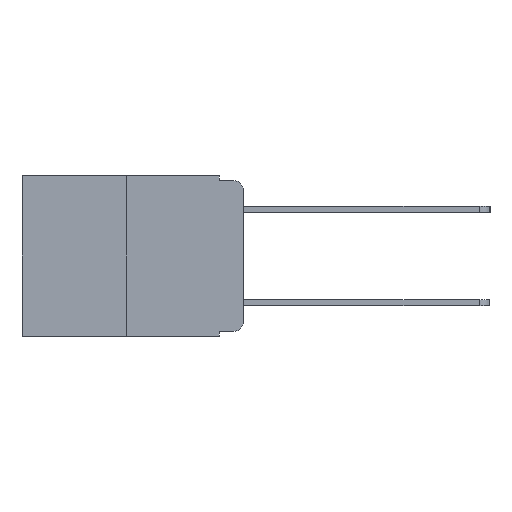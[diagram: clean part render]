
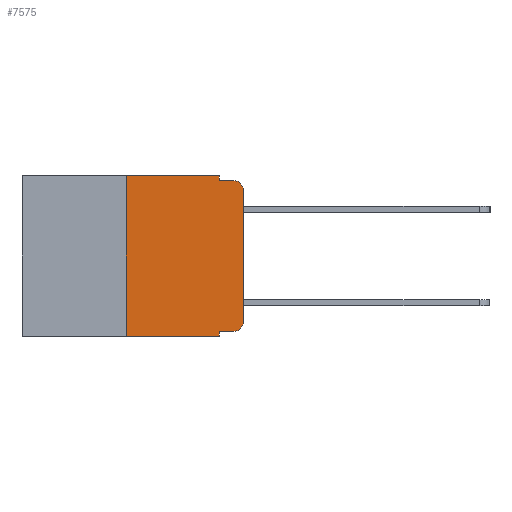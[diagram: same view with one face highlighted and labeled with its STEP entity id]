
A CAD part, left-side view. The second image highlights one B-rep face of the part: STEP entity #7575.
In plain terms, the highlighted planar face has unit normal (-1, 0, 0).
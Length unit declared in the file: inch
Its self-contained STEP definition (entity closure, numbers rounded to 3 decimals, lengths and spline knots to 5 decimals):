
#21 = ORIENTED_EDGE ( 'NONE', *, *, #9780, .F. ) ;
#53 = EDGE_CURVE ( 'NONE', #6673, #9982, #2832, .T. ) ;
#130 = VERTEX_POINT ( 'NONE', #5773 ) ;
#271 = DIRECTION ( 'NONE',  ( 0., 0., 1. ) ) ;
#294 = PLANE ( 'NONE',  #10442 ) ;
#324 = LINE ( 'NONE', #3387, #2792 ) ;
#1171 = DIRECTION ( 'NONE',  ( -1., 0., 0. ) ) ;
#1181 = CARTESIAN_POINT ( 'NONE',  ( 0., 0.02, -0.01 ) ) ;
#1398 = CARTESIAN_POINT ( 'NONE',  ( 0., 0.473, 0. ) ) ;
#1444 = DIRECTION ( 'NONE',  ( 0., 0., -1. ) ) ;
#1502 = CARTESIAN_POINT ( 'NONE',  ( 0., 0.051, -0.343 ) ) ;
#1526 = CARTESIAN_POINT ( 'NONE',  ( 0., 0.25, -0.343 ) ) ;
#1601 = VERTEX_POINT ( 'NONE', #10318 ) ;
#1723 = CARTESIAN_POINT ( 'NONE',  ( 0., 0., -0.313 ) ) ;
#2147 = AXIS2_PLACEMENT_3D ( 'NONE', #6851, #1171, #7711 ) ;
#2165 = CARTESIAN_POINT ( 'NONE',  ( 0., 0.02, -0.313 ) ) ;
#2290 = VECTOR ( 'NONE', #9321, 39.37008 ) ;
#2334 = VERTEX_POINT ( 'NONE', #5200 ) ;
#2429 = DIRECTION ( 'NONE',  ( 0., 0., -1. ) ) ;
#2653 = FACE_OUTER_BOUND ( 'NONE', #3394, .T. ) ;
#2792 = VECTOR ( 'NONE', #271, 39.37008 ) ;
#2832 = LINE ( 'NONE', #11285, #3919 ) ;
#2994 = ORIENTED_EDGE ( 'NONE', *, *, #10386, .T. ) ;
#3154 = DIRECTION ( 'NONE',  ( 0., 0., -1. ) ) ;
#3289 = ORIENTED_EDGE ( 'NONE', *, *, #9850, .T. ) ;
#3387 = CARTESIAN_POINT ( 'NONE',  ( 0., 0.25, 0. ) ) ;
#3394 = EDGE_LOOP ( 'NONE', ( #2994, #3289, #6341, #8844, #21, #4039, #3494, #9813, #10316, #4679 ) ) ;
#3494 = ORIENTED_EDGE ( 'NONE', *, *, #53, .T. ) ;
#3524 = VERTEX_POINT ( 'NONE', #8929 ) ;
#3849 = CARTESIAN_POINT ( 'NONE',  ( 0., 0.473, 0. ) ) ;
#3919 = VECTOR ( 'NONE', #10484, 39.37008 ) ;
#3980 = CARTESIAN_POINT ( 'NONE',  ( 0., 0., 0. ) ) ;
#4039 = ORIENTED_EDGE ( 'NONE', *, *, #8185, .F. ) ;
#4239 = LINE ( 'NONE', #3849, #6384 ) ;
#4679 = ORIENTED_EDGE ( 'NONE', *, *, #6466, .T. ) ;
#4829 = LINE ( 'NONE', #10933, #2290 ) ;
#4880 = VERTEX_POINT ( 'NONE', #11084 ) ;
#4928 = VECTOR ( 'NONE', #11630, 39.37008 ) ;
#5101 = CARTESIAN_POINT ( 'NONE',  ( 0., 0.051, 0. ) ) ;
#5200 = CARTESIAN_POINT ( 'NONE',  ( 0., 0., -0.03 ) ) ;
#5322 = CIRCLE ( 'NONE', #6218, 0.02 ) ;
#5773 = CARTESIAN_POINT ( 'NONE',  ( 0., 0.051, -0.333 ) ) ;
#5828 = CIRCLE ( 'NONE', #2147, 0.02 ) ;
#6218 = AXIS2_PLACEMENT_3D ( 'NONE', #2165, #8504, #3154 ) ;
#6258 = VECTOR ( 'NONE', #8592, 39.37008 ) ;
#6310 = LINE ( 'NONE', #10522, #8564 ) ;
#6341 = ORIENTED_EDGE ( 'NONE', *, *, #9297, .F. ) ;
#6384 = VECTOR ( 'NONE', #10751, 39.37008 ) ;
#6466 = EDGE_CURVE ( 'NONE', #3524, #7777, #5322, .T. ) ;
#6673 = VERTEX_POINT ( 'NONE', #1526 ) ;
#6851 = CARTESIAN_POINT ( 'NONE',  ( 0., 0.02, -0.03 ) ) ;
#7059 = EDGE_CURVE ( 'NONE', #130, #3524, #6310, .T. ) ;
#7344 = LINE ( 'NONE', #3980, #4928 ) ;
#7575 = ADVANCED_FACE ( 'NONE', ( #2653 ), #294, .F. ) ;
#7630 = EDGE_CURVE ( 'NONE', #130, #9982, #11343, .T. ) ;
#7711 = DIRECTION ( 'NONE',  ( 0., 0., -1. ) ) ;
#7777 = VERTEX_POINT ( 'NONE', #1723 ) ;
#7889 = DIRECTION ( 'NONE',  ( 1., 0., 0. ) ) ;
#8185 = EDGE_CURVE ( 'NONE', #6673, #4880, #324, .T. ) ;
#8293 = VERTEX_POINT ( 'NONE', #9691 ) ;
#8504 = DIRECTION ( 'NONE',  ( -1., 0., 0. ) ) ;
#8564 = VECTOR ( 'NONE', #11322, 39.37008 ) ;
#8592 = DIRECTION ( 'NONE',  ( 0., 0., -1. ) ) ;
#8726 = EDGE_CURVE ( 'NONE', #1601, #8293, #9058, .T. ) ;
#8844 = ORIENTED_EDGE ( 'NONE', *, *, #8726, .F. ) ;
#8929 = CARTESIAN_POINT ( 'NONE',  ( 0., 0.02, -0.333 ) ) ;
#9058 = LINE ( 'NONE', #5101, #6258 ) ;
#9217 = VECTOR ( 'NONE', #1444, 39.37008 ) ;
#9297 = EDGE_CURVE ( 'NONE', #8293, #9339, #4829, .T. ) ;
#9321 = DIRECTION ( 'NONE',  ( 0., -1., 0. ) ) ;
#9339 = VERTEX_POINT ( 'NONE', #1181 ) ;
#9691 = CARTESIAN_POINT ( 'NONE',  ( 0., 0.051, -0.01 ) ) ;
#9780 = EDGE_CURVE ( 'NONE', #4880, #1601, #4239, .T. ) ;
#9813 = ORIENTED_EDGE ( 'NONE', *, *, #7630, .F. ) ;
#9850 = EDGE_CURVE ( 'NONE', #2334, #9339, #5828, .T. ) ;
#9982 = VERTEX_POINT ( 'NONE', #1502 ) ;
#10316 = ORIENTED_EDGE ( 'NONE', *, *, #7059, .T. ) ;
#10318 = CARTESIAN_POINT ( 'NONE',  ( 0., 0.051, 0. ) ) ;
#10386 = EDGE_CURVE ( 'NONE', #7777, #2334, #7344, .T. ) ;
#10442 = AXIS2_PLACEMENT_3D ( 'NONE', #1398, #7889, #2429 ) ;
#10484 = DIRECTION ( 'NONE',  ( 0., -1., 0. ) ) ;
#10522 = CARTESIAN_POINT ( 'NONE',  ( 0., 0.051, -0.333 ) ) ;
#10751 = DIRECTION ( 'NONE',  ( 0., -1., 0. ) ) ;
#10933 = CARTESIAN_POINT ( 'NONE',  ( 0., 0.051, -0.01 ) ) ;
#11084 = CARTESIAN_POINT ( 'NONE',  ( 0., 0.25, 0. ) ) ;
#11194 = CARTESIAN_POINT ( 'NONE',  ( 0., 0.051, 0. ) ) ;
#11285 = CARTESIAN_POINT ( 'NONE',  ( 0., 0.473, -0.343 ) ) ;
#11322 = DIRECTION ( 'NONE',  ( 0., -1., 0. ) ) ;
#11343 = LINE ( 'NONE', #11194, #9217 ) ;
#11630 = DIRECTION ( 'NONE',  ( 0., 0., 1. ) ) ;
